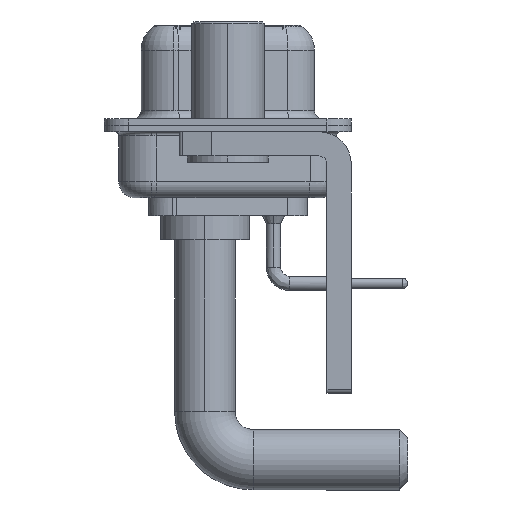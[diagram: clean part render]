
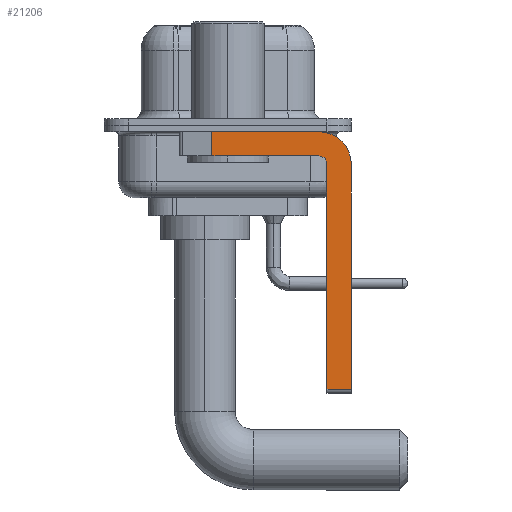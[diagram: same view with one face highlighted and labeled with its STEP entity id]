
A CAD part, left-side view. The second image highlights one B-rep face of the part: STEP entity #21206.
In plain terms, the highlighted planar face has unit normal (-1, 0, 0).
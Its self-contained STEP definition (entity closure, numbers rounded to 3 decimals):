
#118 = ORIENTED_EDGE ( 'NONE', *, *, #16846, .F. ) ;
#391 = VERTEX_POINT ( 'NONE', #20152 ) ;
#505 = VECTOR ( 'NONE', #14109, 1000. ) ;
#651 = DIRECTION ( 'NONE',  ( 0., 0., 1. ) ) ;
#711 = ORIENTED_EDGE ( 'NONE', *, *, #16050, .T. ) ;
#820 = ORIENTED_EDGE ( 'NONE', *, *, #19547, .F. ) ;
#1379 = EDGE_CURVE ( 'NONE', #23247, #4173, #3932, .T. ) ;
#1611 = DIRECTION ( 'NONE',  ( 0., 0., -1. ) ) ;
#1807 = VECTOR ( 'NONE', #18710, 1000. ) ;
#2002 = AXIS2_PLACEMENT_3D ( 'NONE', #2339, #17096, #651 ) ;
#2174 = VECTOR ( 'NONE', #4397, 1000. ) ;
#2339 = CARTESIAN_POINT ( 'NONE',  ( -2.9, -5.65, -2.4 ) ) ;
#3262 = CARTESIAN_POINT ( 'NONE',  ( -2.9, -7.65, -2.4 ) ) ;
#3932 = CIRCLE ( 'NONE', #2002, 0.5 ) ;
#4173 = VERTEX_POINT ( 'NONE', #4690 ) ;
#4362 = AXIS2_PLACEMENT_3D ( 'NONE', #13971, #8933, #21293 ) ;
#4397 = DIRECTION ( 'NONE',  ( 0., 1., 0. ) ) ;
#4690 = CARTESIAN_POINT ( 'NONE',  ( -2.9, -5.65, -1.9 ) ) ;
#4913 = ORIENTED_EDGE ( 'NONE', *, *, #1379, .F. ) ;
#4922 = CARTESIAN_POINT ( 'NONE',  ( -2.9, 0.978, -1.9 ) ) ;
#5108 = EDGE_CURVE ( 'NONE', #21618, #391, #17677, .T. ) ;
#5243 = VERTEX_POINT ( 'NONE', #19699 ) ;
#5303 = CIRCLE ( 'NONE', #12183, 2. ) ;
#5674 = CARTESIAN_POINT ( 'NONE',  ( -2.9, -6.15, -2.4 ) ) ;
#5852 = CARTESIAN_POINT ( 'NONE',  ( -2.9, -6.15, -16.35 ) ) ;
#6407 = CARTESIAN_POINT ( 'NONE',  ( -2.9, -7.65, -2.4 ) ) ;
#6528 = ORIENTED_EDGE ( 'NONE', *, *, #5108, .F. ) ;
#6737 = ORIENTED_EDGE ( 'NONE', *, *, #14462, .T. ) ;
#6814 = LINE ( 'NONE', #21436, #505 ) ;
#7272 = CARTESIAN_POINT ( 'NONE',  ( -2.9, -5.65, -2.4 ) ) ;
#7937 = VERTEX_POINT ( 'NONE', #5852 ) ;
#8447 = DIRECTION ( 'NONE',  ( 0., 0., -1. ) ) ;
#8553 = DIRECTION ( 'NONE',  ( 0., 0., 1. ) ) ;
#8933 = DIRECTION ( 'NONE',  ( 1., 0., 0. ) ) ;
#9022 = CARTESIAN_POINT ( 'NONE',  ( -2.9, -6.15, -16.6 ) ) ;
#9350 = LINE ( 'NONE', #22541, #1807 ) ;
#9789 = EDGE_LOOP ( 'NONE', ( #820, #6737, #21125, #4913, #11106, #711, #6528, #118 ) ) ;
#9977 = LINE ( 'NONE', #10207, #18344 ) ;
#10207 = CARTESIAN_POINT ( 'NONE',  ( -2.9, -5.65, -16.35 ) ) ;
#10750 = PLANE ( 'NONE',  #4362 ) ;
#10992 = DIRECTION ( 'NONE',  ( 1., 0., 0. ) ) ;
#11106 = ORIENTED_EDGE ( 'NONE', *, *, #15787, .F. ) ;
#12183 = AXIS2_PLACEMENT_3D ( 'NONE', #7272, #10992, #1611 ) ;
#12941 = VERTEX_POINT ( 'NONE', #4922 ) ;
#13504 = CARTESIAN_POINT ( 'NONE',  ( -2.9, -5.65, -1.9 ) ) ;
#13784 = EDGE_CURVE ( 'NONE', #4173, #12941, #17466, .T. ) ;
#13971 = CARTESIAN_POINT ( 'NONE',  ( -2.9, -5.65, -2.4 ) ) ;
#14109 = DIRECTION ( 'NONE',  ( 0., -1., 0. ) ) ;
#14115 = VECTOR ( 'NONE', #8553, 1000. ) ;
#14462 = EDGE_CURVE ( 'NONE', #14504, #12941, #9350, .T. ) ;
#14504 = VERTEX_POINT ( 'NONE', #18826 ) ;
#15787 = EDGE_CURVE ( 'NONE', #7937, #23247, #18025, .T. ) ;
#16050 = EDGE_CURVE ( 'NONE', #7937, #391, #9977, .T. ) ;
#16846 = EDGE_CURVE ( 'NONE', #5243, #21618, #5303, .T. ) ;
#17055 = VECTOR ( 'NONE', #8447, 1000. ) ;
#17096 = DIRECTION ( 'NONE',  ( -1., 0., 0. ) ) ;
#17466 = LINE ( 'NONE', #13504, #2174 ) ;
#17525 = DIRECTION ( 'NONE',  ( 0., -1., 0. ) ) ;
#17677 = LINE ( 'NONE', #6407, #17055 ) ;
#17942 = FACE_OUTER_BOUND ( 'NONE', #9789, .T. ) ;
#18025 = LINE ( 'NONE', #9022, #14115 ) ;
#18344 = VECTOR ( 'NONE', #17525, 1000. ) ;
#18710 = DIRECTION ( 'NONE',  ( 0., 0., -1. ) ) ;
#18826 = CARTESIAN_POINT ( 'NONE',  ( -2.9, 0.978, -0.4 ) ) ;
#19547 = EDGE_CURVE ( 'NONE', #14504, #5243, #6814, .T. ) ;
#19699 = CARTESIAN_POINT ( 'NONE',  ( -2.9, -5.65, -0.4 ) ) ;
#20152 = CARTESIAN_POINT ( 'NONE',  ( -2.9, -7.65, -16.35 ) ) ;
#21125 = ORIENTED_EDGE ( 'NONE', *, *, #13784, .F. ) ;
#21206 = ADVANCED_FACE ( 'NONE', ( #17942 ), #10750, .F. ) ;
#21293 = DIRECTION ( 'NONE',  ( 0., 0., -1. ) ) ;
#21436 = CARTESIAN_POINT ( 'NONE',  ( -2.9, 3., -0.4 ) ) ;
#21618 = VERTEX_POINT ( 'NONE', #3262 ) ;
#22541 = CARTESIAN_POINT ( 'NONE',  ( -2.9, 0.978, -1.9 ) ) ;
#23247 = VERTEX_POINT ( 'NONE', #5674 ) ;
